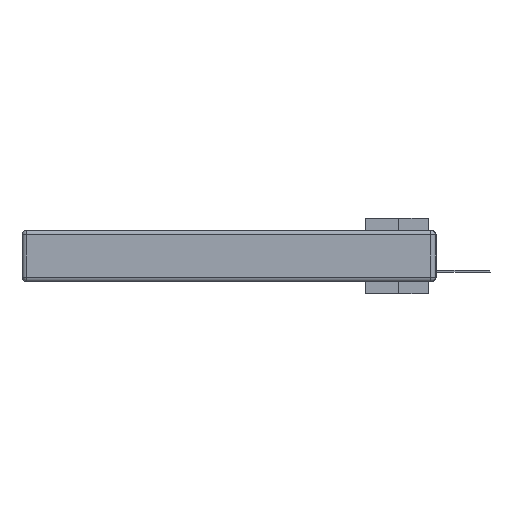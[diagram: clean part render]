
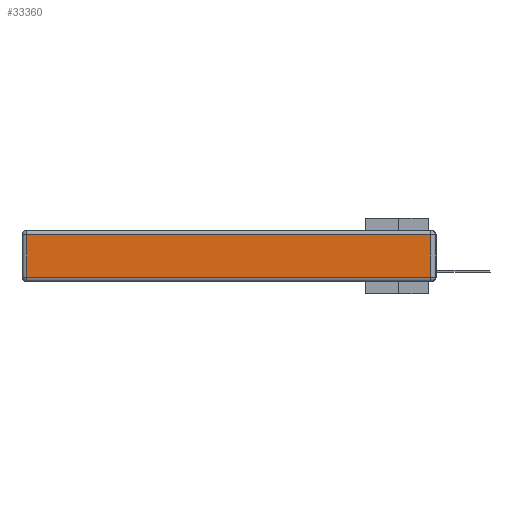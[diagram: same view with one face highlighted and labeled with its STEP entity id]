
A CAD part, left-side view. The second image highlights one B-rep face of the part: STEP entity #33360.
In plain terms, the highlighted planar face has unit normal (-1, 0, 0).
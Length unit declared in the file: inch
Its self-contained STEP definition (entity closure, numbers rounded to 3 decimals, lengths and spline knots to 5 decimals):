
#1541 = EDGE_CURVE ( 'NONE', #19292, #8061, #9193, .T. ) ;
#3099 = DIRECTION ( 'NONE',  ( 0., 0., -1. ) ) ;
#3518 = VECTOR ( 'NONE', #11439, 39.37008 ) ;
#3576 = DIRECTION ( 'NONE',  ( 0., 1., 0. ) ) ;
#4974 = PLANE ( 'NONE',  #13766 ) ;
#5918 = CARTESIAN_POINT ( 'NONE',  ( 0., 2.72, -0.343 ) ) ;
#8061 = VERTEX_POINT ( 'NONE', #21636 ) ;
#9193 = LINE ( 'NONE', #30393, #33137 ) ;
#9656 = LINE ( 'NONE', #5918, #27013 ) ;
#10431 = DIRECTION ( 'NONE',  ( 0., 0., 1. ) ) ;
#11296 = VERTEX_POINT ( 'NONE', #27315 ) ;
#11439 = DIRECTION ( 'NONE',  ( 0., 0., 1. ) ) ;
#12728 = ORIENTED_EDGE ( 'NONE', *, *, #28460, .T. ) ;
#12847 = DIRECTION ( 'NONE',  ( -1., 0., 0. ) ) ;
#13766 = AXIS2_PLACEMENT_3D ( 'NONE', #28327, #12847, #10431 ) ;
#15055 = ORIENTED_EDGE ( 'NONE', *, *, #26764, .T. ) ;
#15225 = EDGE_CURVE ( 'NONE', #8061, #11296, #9656, .T. ) ;
#15988 = CARTESIAN_POINT ( 'NONE',  ( 0., 0., -0.313 ) ) ;
#19102 = ORIENTED_EDGE ( 'NONE', *, *, #15225, .T. ) ;
#19292 = VERTEX_POINT ( 'NONE', #31752 ) ;
#21282 = ORIENTED_EDGE ( 'NONE', *, *, #1541, .T. ) ;
#21636 = CARTESIAN_POINT ( 'NONE',  ( 0., 2.72, -0.03 ) ) ;
#22032 = FACE_OUTER_BOUND ( 'NONE', #27814, .T. ) ;
#23286 = LINE ( 'NONE', #15988, #27730 ) ;
#23397 = LINE ( 'NONE', #29401, #3518 ) ;
#24749 = CARTESIAN_POINT ( 'NONE',  ( 0., 0.03, -0.313 ) ) ;
#26026 = DIRECTION ( 'NONE',  ( 0., -1., 0. ) ) ;
#26764 = EDGE_CURVE ( 'NONE', #32427, #19292, #23397, .T. ) ;
#27013 = VECTOR ( 'NONE', #3099, 39.37008 ) ;
#27315 = CARTESIAN_POINT ( 'NONE',  ( 0., 2.72, -0.313 ) ) ;
#27730 = VECTOR ( 'NONE', #26026, 39.37008 ) ;
#27814 = EDGE_LOOP ( 'NONE', ( #12728, #15055, #21282, #19102 ) ) ;
#28327 = CARTESIAN_POINT ( 'NONE',  ( 0., 0., -0.343 ) ) ;
#28460 = EDGE_CURVE ( 'NONE', #11296, #32427, #23286, .T. ) ;
#29401 = CARTESIAN_POINT ( 'NONE',  ( 0., 0.03, -0.343 ) ) ;
#30393 = CARTESIAN_POINT ( 'NONE',  ( 0., 2.75, -0.03 ) ) ;
#31752 = CARTESIAN_POINT ( 'NONE',  ( 0., 0.03, -0.03 ) ) ;
#32427 = VERTEX_POINT ( 'NONE', #24749 ) ;
#33137 = VECTOR ( 'NONE', #3576, 39.37008 ) ;
#33360 = ADVANCED_FACE ( 'NONE', ( #22032 ), #4974, .T. ) ;
